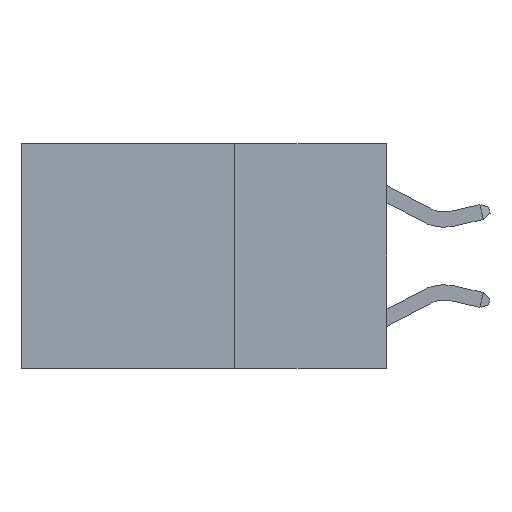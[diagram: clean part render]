
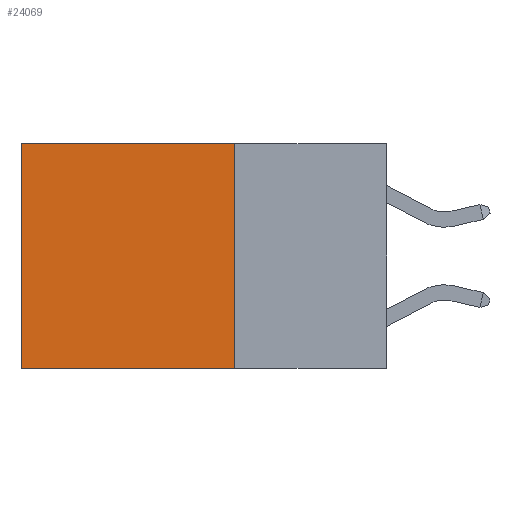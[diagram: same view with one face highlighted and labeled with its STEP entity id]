
A CAD part, left-side view. The second image highlights one B-rep face of the part: STEP entity #24069.
In plain terms, the highlighted planar face has unit normal (-1, 0, 0).
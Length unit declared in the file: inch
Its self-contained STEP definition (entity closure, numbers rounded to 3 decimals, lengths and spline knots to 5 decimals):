
#2664 = LINE ( 'NONE', #29201, #26834 ) ;
#3554 = DIRECTION ( 'NONE',  ( 0., 0., -1. ) ) ;
#4199 = ORIENTED_EDGE ( 'NONE', *, *, #24251, .T. ) ;
#4333 = AXIS2_PLACEMENT_3D ( 'NONE', #19741, #17227, #28913 ) ;
#5004 = CARTESIAN_POINT ( 'NONE',  ( 0.2625, 0.6, 0. ) ) ;
#7606 = FACE_OUTER_BOUND ( 'NONE', #12352, .T. ) ;
#11379 = EDGE_CURVE ( 'NONE', #12599, #23599, #24452, .T. ) ;
#12352 = EDGE_LOOP ( 'NONE', ( #4199, #27030, #25397, #15819 ) ) ;
#12599 = VERTEX_POINT ( 'NONE', #16900 ) ;
#13791 = VECTOR ( 'NONE', #29338, 39.37008 ) ;
#14438 = CARTESIAN_POINT ( 'NONE',  ( 0.2625, 0.25, -0.37 ) ) ;
#14668 = CARTESIAN_POINT ( 'NONE',  ( 0.2625, 0.25, 0. ) ) ;
#15217 = CARTESIAN_POINT ( 'NONE',  ( 0.2625, 0.6, -0.37 ) ) ;
#15781 = CARTESIAN_POINT ( 'NONE',  ( 0.2625, 0.6, 0. ) ) ;
#15819 = ORIENTED_EDGE ( 'NONE', *, *, #11379, .T. ) ;
#16793 = VERTEX_POINT ( 'NONE', #15217 ) ;
#16900 = CARTESIAN_POINT ( 'NONE',  ( 0.2625, 0.25, 0. ) ) ;
#17227 = DIRECTION ( 'NONE',  ( 1., 0., 0. ) ) ;
#17541 = PLANE ( 'NONE',  #4333 ) ;
#19741 = CARTESIAN_POINT ( 'NONE',  ( 0.2625, 0.25, 0. ) ) ;
#20376 = EDGE_CURVE ( 'NONE', #12599, #20572, #23128, .T. ) ;
#20572 = VERTEX_POINT ( 'NONE', #14438 ) ;
#20674 = LINE ( 'NONE', #15781, #24490 ) ;
#22089 = DIRECTION ( 'NONE',  ( 0., 1., 0. ) ) ;
#23128 = LINE ( 'NONE', #23286, #24405 ) ;
#23286 = CARTESIAN_POINT ( 'NONE',  ( 0.2625, 0.25, 0. ) ) ;
#23599 = VERTEX_POINT ( 'NONE', #5004 ) ;
#24069 = ADVANCED_FACE ( 'NONE', ( #7606 ), #17541, .F. ) ;
#24251 = EDGE_CURVE ( 'NONE', #23599, #16793, #20674, .T. ) ;
#24405 = VECTOR ( 'NONE', #3554, 39.37008 ) ;
#24452 = LINE ( 'NONE', #14668, #13791 ) ;
#24490 = VECTOR ( 'NONE', #25417, 39.37008 ) ;
#25397 = ORIENTED_EDGE ( 'NONE', *, *, #20376, .F. ) ;
#25417 = DIRECTION ( 'NONE',  ( 0., 0., -1. ) ) ;
#26834 = VECTOR ( 'NONE', #22089, 39.37008 ) ;
#27030 = ORIENTED_EDGE ( 'NONE', *, *, #29880, .F. ) ;
#28913 = DIRECTION ( 'NONE',  ( 0., 0., -1. ) ) ;
#29201 = CARTESIAN_POINT ( 'NONE',  ( 0.2625, 0.25, -0.37 ) ) ;
#29338 = DIRECTION ( 'NONE',  ( 0., 1., 0. ) ) ;
#29880 = EDGE_CURVE ( 'NONE', #20572, #16793, #2664, .T. ) ;
